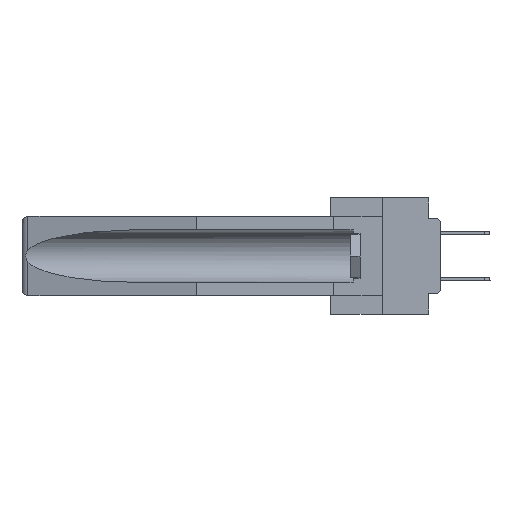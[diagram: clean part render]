
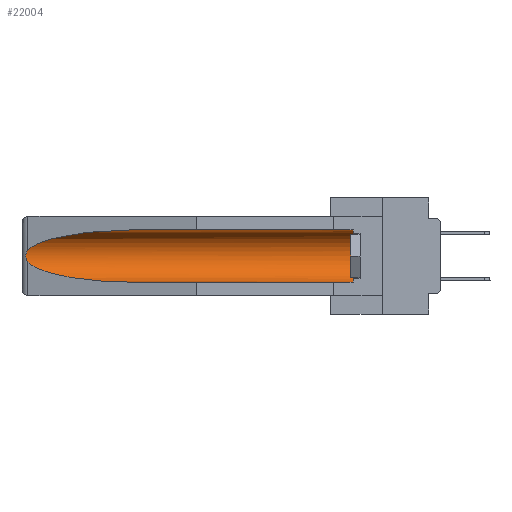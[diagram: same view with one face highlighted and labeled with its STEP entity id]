
A CAD part, left-side view. The second image highlights one B-rep face of the part: STEP entity #22004.
In plain terms, the highlighted cylindrical face has radius 2.857 mm (diameter 5.715 mm), a partial arc.
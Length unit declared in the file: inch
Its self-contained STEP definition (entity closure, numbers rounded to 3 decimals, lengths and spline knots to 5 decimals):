
#438 = DIRECTION ( 'NONE',  ( 0., 1., 0. ) ) ;
#1129 = CARTESIAN_POINT ( 'NONE',  ( 0.26597, 1.52961, -0.15275 ) ) ;
#1330 = CARTESIAN_POINT ( 'NONE',  ( 0.2675, 1.53308, -0.16763 ) ) ;
#1386 = EDGE_CURVE ( 'NONE', #7329, #35442, #10728, .T. ) ;
#1483 = DIRECTION ( 'NONE',  ( 0., 0., 1. ) ) ;
#1534 = CARTESIAN_POINT ( 'NONE',  ( 0.2673, 1.53269, -0.17917 ) ) ;
#3410 = LINE ( 'NONE', #6178, #19734 ) ;
#4240 = CARTESIAN_POINT ( 'NONE',  ( 0.21114, 1.30732, -0.059 ) ) ;
#4290 = CARTESIAN_POINT ( 'NONE',  ( 0.2673, 1.5327, -0.16383 ) ) ;
#4440 = CARTESIAN_POINT ( 'NONE',  ( 0.25451, 1.48313, -0.09465 ) ) ;
#4702 = CARTESIAN_POINT ( 'NONE',  ( 0.2675, 1.53308, -0.17534 ) ) ;
#5037 = ORIENTED_EDGE ( 'NONE', *, *, #14061, .F. ) ;
#5285 = ORIENTED_EDGE ( 'NONE', *, *, #8135, .T. ) ;
#6178 = CARTESIAN_POINT ( 'NONE',  ( 0.155, -0.30754, -0.059 ) ) ;
#6858 = CARTESIAN_POINT ( 'NONE',  ( 0.26655, 1.53094, -0.18657 ) ) ;
#7329 = VERTEX_POINT ( 'NONE', #9811 ) ;
#8135 = EDGE_CURVE ( 'NONE', #35442, #30806, #9557, .T. ) ;
#8413 = EDGE_CURVE ( 'NONE', #12708, #8764, #29724, .T. ) ;
#8764 = VERTEX_POINT ( 'NONE', #33654 ) ;
#9211 = ORIENTED_EDGE ( 'NONE', *, *, #8413, .T. ) ;
#9398 = EDGE_CURVE ( 'NONE', #30806, #25824, #21797, .T. ) ;
#9557 = B_SPLINE_CURVE_WITH_KNOTS ( 'NONE', 3,
 ( #34513, #1129, #34712, #4290, #1330, #4702, #1534, #6858, #13407, #34134 ),
 .UNSPECIFIED., .F., .F.,
 ( 4, 2, 2, 2, 4 ),
 ( 0., 0.00029, 0.00058, 0.00087, 0.00117 ),
 .UNSPECIFIED. ) ;
#9811 = CARTESIAN_POINT ( 'NONE',  ( 0.155, 1.07973, -0.059 ) ) ;
#10384 = CARTESIAN_POINT ( 'NONE',  ( 0.155, -0.30754, -0.1715 ) ) ;
#10728 =( BOUNDED_CURVE ( )  B_SPLINE_CURVE ( 3, ( #31327, #4240, #4440, #13363 ),
 .UNSPECIFIED., .F., .F. ) 
 B_SPLINE_CURVE_WITH_KNOTS ( ( 4, 4 ),
 ( 4.71239, 6.08839 ),
 .UNSPECIFIED. ) 
 CURVE ( )  GEOMETRIC_REPRESENTATION_ITEM ( )  RATIONAL_B_SPLINE_CURVE ( ( 1., 0.848, 0.848, 1. ) ) 
 REPRESENTATION_ITEM ( '' )  );
#12091 = CARTESIAN_POINT ( 'NONE',  ( 0.155, 1.07973, -0.284 ) ) ;
#12196 = DIRECTION ( 'NONE',  ( 0., 0., 1. ) ) ;
#12216 = VECTOR ( 'NONE', #25192, 39.37008 ) ;
#12708 = VERTEX_POINT ( 'NONE', #30545 ) ;
#12974 = CARTESIAN_POINT ( 'NONE',  ( 0.155, -0.30754, -0.284 ) ) ;
#13363 = CARTESIAN_POINT ( 'NONE',  ( 0.26537, 1.52718, -0.14972 ) ) ;
#13407 = CARTESIAN_POINT ( 'NONE',  ( 0.26597, 1.5296, -0.19026 ) ) ;
#13758 = LINE ( 'NONE', #12974, #12216 ) ;
#14061 = EDGE_CURVE ( 'NONE', #12708, #25824, #13758, .T. ) ;
#14611 = AXIS2_PLACEMENT_3D ( 'NONE', #24593, #29976, #12196 ) ;
#15514 = ORIENTED_EDGE ( 'NONE', *, *, #1386, .T. ) ;
#16915 = FACE_OUTER_BOUND ( 'NONE', #22398, .T. ) ;
#19514 = CARTESIAN_POINT ( 'NONE',  ( 0.155, 1.07973, -0.284 ) ) ;
#19734 = VECTOR ( 'NONE', #438, 39.37008 ) ;
#20179 = CARTESIAN_POINT ( 'NONE',  ( 0.26537, 1.52718, -0.19328 ) ) ;
#20797 = ORIENTED_EDGE ( 'NONE', *, *, #9398, .T. ) ;
#20982 = EDGE_CURVE ( 'NONE', #8764, #7329, #3410, .T. ) ;
#21431 = AXIS2_PLACEMENT_3D ( 'NONE', #10384, #32117, #1483 ) ;
#21797 =( BOUNDED_CURVE ( )  B_SPLINE_CURVE ( 3, ( #31374, #31973, #22492, #19514 ),
 .UNSPECIFIED., .F., .F. ) 
 B_SPLINE_CURVE_WITH_KNOTS ( ( 4, 4 ),
 ( 0.1948, 1.5708 ),
 .UNSPECIFIED. ) 
 CURVE ( )  GEOMETRIC_REPRESENTATION_ITEM ( )  RATIONAL_B_SPLINE_CURVE ( ( 1., 0.848, 0.848, 1. ) ) 
 REPRESENTATION_ITEM ( '' )  );
#22004 = ADVANCED_FACE ( 'NONE', ( #16915 ), #23031, .F. ) ;
#22398 = EDGE_LOOP ( 'NONE', ( #15514, #5285, #20797, #5037, #9211, #23913 ) ) ;
#22492 = CARTESIAN_POINT ( 'NONE',  ( 0.21114, 1.30732, -0.284 ) ) ;
#23031 = CYLINDRICAL_SURFACE ( 'NONE', #21431, 0.1125 ) ;
#23913 = ORIENTED_EDGE ( 'NONE', *, *, #20982, .T. ) ;
#24593 = CARTESIAN_POINT ( 'NONE',  ( 0.155, 0.126, -0.1715 ) ) ;
#25192 = DIRECTION ( 'NONE',  ( 0., 1., 0. ) ) ;
#25824 = VERTEX_POINT ( 'NONE', #12091 ) ;
#29724 = CIRCLE ( 'NONE', #14611, 0.1125 ) ;
#29976 = DIRECTION ( 'NONE',  ( 0., -1., 0. ) ) ;
#30545 = CARTESIAN_POINT ( 'NONE',  ( 0.155, 0.126, -0.284 ) ) ;
#30806 = VERTEX_POINT ( 'NONE', #20179 ) ;
#31327 = CARTESIAN_POINT ( 'NONE',  ( 0.155, 1.07973, -0.059 ) ) ;
#31374 = CARTESIAN_POINT ( 'NONE',  ( 0.26537, 1.52718, -0.19328 ) ) ;
#31973 = CARTESIAN_POINT ( 'NONE',  ( 0.25451, 1.48313, -0.24835 ) ) ;
#32117 = DIRECTION ( 'NONE',  ( 0., 1., 0. ) ) ;
#33654 = CARTESIAN_POINT ( 'NONE',  ( 0.155, 0.126, -0.059 ) ) ;
#34134 = CARTESIAN_POINT ( 'NONE',  ( 0.26537, 1.52718, -0.19328 ) ) ;
#34232 = CARTESIAN_POINT ( 'NONE',  ( 0.26537, 1.52718, -0.14972 ) ) ;
#34513 = CARTESIAN_POINT ( 'NONE',  ( 0.26537, 1.52718, -0.14972 ) ) ;
#34712 = CARTESIAN_POINT ( 'NONE',  ( 0.26654, 1.53092, -0.15636 ) ) ;
#35442 = VERTEX_POINT ( 'NONE', #34232 ) ;
